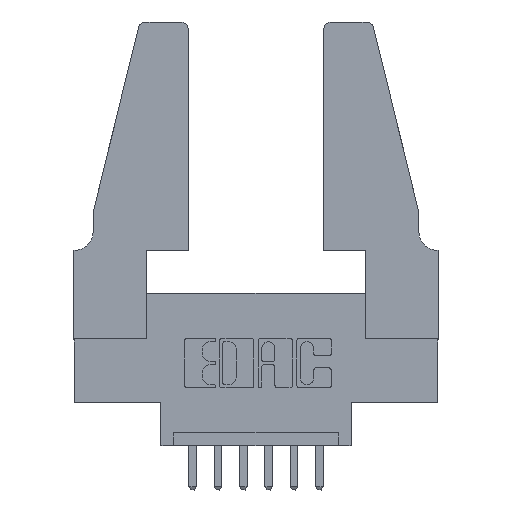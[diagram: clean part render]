
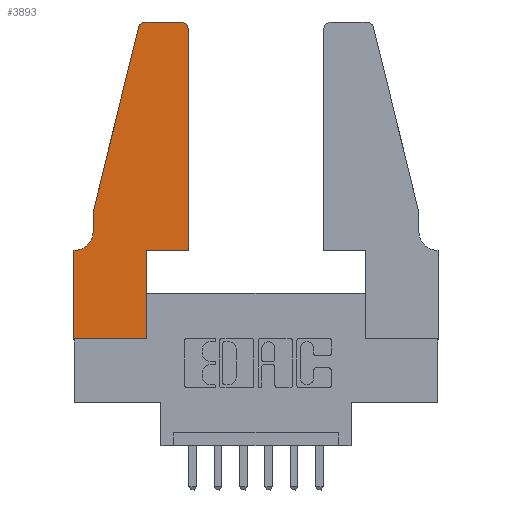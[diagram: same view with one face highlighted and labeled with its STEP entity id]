
A CAD part, top view. The second image highlights one B-rep face of the part: STEP entity #3893.
In plain terms, the highlighted planar face has unit normal (0, 0, 1).
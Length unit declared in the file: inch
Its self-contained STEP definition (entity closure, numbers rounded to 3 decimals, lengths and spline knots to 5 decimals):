
#195 = ORIENTED_EDGE ( 'NONE', *, *, #6748, .T. ) ;
#251 = AXIS2_PLACEMENT_3D ( 'NONE', #9541, #4079, #5767 ) ;
#274 = LINE ( 'NONE', #6401, #10389 ) ;
#316 = CARTESIAN_POINT ( 'NONE',  ( 0., 0., 0.37 ) ) ;
#455 = ORIENTED_EDGE ( 'NONE', *, *, #7087, .T. ) ;
#962 = EDGE_CURVE ( 'NONE', #7101, #1618, #11481, .T. ) ;
#1099 = CARTESIAN_POINT ( 'NONE',  ( 0.4505, 1.22, 0.37 ) ) ;
#1188 = ORIENTED_EDGE ( 'NONE', *, *, #3649, .T. ) ;
#1441 = VERTEX_POINT ( 'NONE', #6241 ) ;
#1507 = ORIENTED_EDGE ( 'NONE', *, *, #8306, .T. ) ;
#1570 = VECTOR ( 'NONE', #3611, 39.37008 ) ;
#1574 = DIRECTION ( 'NONE',  ( 1., 0., 0. ) ) ;
#1618 = VERTEX_POINT ( 'NONE', #7094 ) ;
#1653 = DIRECTION ( 'NONE',  ( -1., 0., 0. ) ) ;
#1662 = DIRECTION ( 'NONE',  ( 0., -1., 0. ) ) ;
#1713 = DIRECTION ( 'NONE',  ( 1., 0., 0. ) ) ;
#1851 = CARTESIAN_POINT ( 'NONE',  ( 0.0055, 0.35, 0.37 ) ) ;
#1860 = VECTOR ( 'NONE', #10426, 39.37008 ) ;
#1876 = ORIENTED_EDGE ( 'NONE', *, *, #962, .T. ) ;
#2293 = DIRECTION ( 'NONE',  ( 0., 0., -1. ) ) ;
#2810 = EDGE_CURVE ( 'NONE', #6537, #9482, #8172, .T. ) ;
#2836 = DIRECTION ( 'NONE',  ( 0., 1., 0. ) ) ;
#2928 = AXIS2_PLACEMENT_3D ( 'NONE', #3253, #2293, #9629 ) ;
#3149 = EDGE_CURVE ( 'NONE', #3715, #5302, #3883, .T. ) ;
#3253 = CARTESIAN_POINT ( 'NONE',  ( 0.0055, 0.42, 0.37 ) ) ;
#3288 = ORIENTED_EDGE ( 'NONE', *, *, #3149, .T. ) ;
#3290 = VERTEX_POINT ( 'NONE', #11260 ) ;
#3559 = CIRCLE ( 'NONE', #251, 0.03 ) ;
#3611 = DIRECTION ( 'NONE',  ( 1., 0., 0. ) ) ;
#3649 = EDGE_CURVE ( 'NONE', #5302, #11362, #4439, .T. ) ;
#3688 = VERTEX_POINT ( 'NONE', #9866 ) ;
#3715 = VERTEX_POINT ( 'NONE', #1851 ) ;
#3883 = LINE ( 'NONE', #7108, #10729 ) ;
#3893 = ADVANCED_FACE ( 'NONE', ( #6840 ), #5162, .T. ) ;
#3998 = VECTOR ( 'NONE', #1662, 39.37008 ) ;
#4022 = AXIS2_PLACEMENT_3D ( 'NONE', #5936, #10556, #6027 ) ;
#4079 = DIRECTION ( 'NONE',  ( 0., 0., 1. ) ) ;
#4189 = EDGE_CURVE ( 'NONE', #3290, #6929, #10902, .T. ) ;
#4343 = VERTEX_POINT ( 'NONE', #10335 ) ;
#4439 = LINE ( 'NONE', #6169, #3998 ) ;
#4602 = ORIENTED_EDGE ( 'NONE', *, *, #9904, .T. ) ;
#4687 = LINE ( 'NONE', #9246, #1860 ) ;
#5062 = LINE ( 'NONE', #6744, #11759 ) ;
#5162 = PLANE ( 'NONE',  #8461 ) ;
#5298 = CARTESIAN_POINT ( 'NONE',  ( 0., 0.35, 0.37 ) ) ;
#5302 = VERTEX_POINT ( 'NONE', #5298 ) ;
#5452 = ORIENTED_EDGE ( 'NONE', *, *, #4189, .T. ) ;
#5462 = CARTESIAN_POINT ( 'NONE',  ( 0.0755, 0.5, 0.37 ) ) ;
#5469 = CIRCLE ( 'NONE', #2928, 0.07 ) ;
#5507 = VECTOR ( 'NONE', #1713, 39.37008 ) ;
#5767 = DIRECTION ( 'NONE',  ( 1., 0., 0. ) ) ;
#5805 = LINE ( 'NONE', #7338, #1570 ) ;
#5930 = CARTESIAN_POINT ( 'NONE',  ( 0.4205, 1.25, 0.37 ) ) ;
#5936 = CARTESIAN_POINT ( 'NONE',  ( 0.4205, 1.22, 0.37 ) ) ;
#6002 = ORIENTED_EDGE ( 'NONE', *, *, #7707, .T. ) ;
#6027 = DIRECTION ( 'NONE',  ( 1., 0., 0. ) ) ;
#6089 = CARTESIAN_POINT ( 'NONE',  ( 0., 0.35, 0.37 ) ) ;
#6169 = CARTESIAN_POINT ( 'NONE',  ( 0., 0., 0.37 ) ) ;
#6241 = CARTESIAN_POINT ( 'NONE',  ( 0.284, 1.25, 0.37 ) ) ;
#6345 = ORIENTED_EDGE ( 'NONE', *, *, #2810, .T. ) ;
#6401 = CARTESIAN_POINT ( 'NONE',  ( 0.2605, 1.25, 0.37 ) ) ;
#6537 = VERTEX_POINT ( 'NONE', #1099 ) ;
#6744 = CARTESIAN_POINT ( 'NONE',  ( 0.0755, 0.5, 0.37 ) ) ;
#6748 = EDGE_CURVE ( 'NONE', #1441, #3688, #3559, .T. ) ;
#6840 = FACE_OUTER_BOUND ( 'NONE', #11246, .T. ) ;
#6929 = VERTEX_POINT ( 'NONE', #8174 ) ;
#7087 = EDGE_CURVE ( 'NONE', #4343, #6537, #4687, .T. ) ;
#7094 = CARTESIAN_POINT ( 'NONE',  ( 0.0755, 0.42, 0.37 ) ) ;
#7101 = VERTEX_POINT ( 'NONE', #8583 ) ;
#7108 = CARTESIAN_POINT ( 'NONE',  ( 0.0755, 0.35, 0.37 ) ) ;
#7211 = ORIENTED_EDGE ( 'NONE', *, *, #9388, .T. ) ;
#7338 = CARTESIAN_POINT ( 'NONE',  ( 0.4505, 0.35, 0.37 ) ) ;
#7401 = DIRECTION ( 'NONE',  ( -1., 0., 0. ) ) ;
#7696 = DIRECTION ( 'NONE',  ( -0.239, -0.971, 0. ) ) ;
#7707 = EDGE_CURVE ( 'NONE', #6929, #4343, #5805, .T. ) ;
#7888 = EDGE_CURVE ( 'NONE', #9482, #1441, #274, .T. ) ;
#8172 = CIRCLE ( 'NONE', #4022, 0.03 ) ;
#8174 = CARTESIAN_POINT ( 'NONE',  ( 0.2865, 0.35, 0.37 ) ) ;
#8306 = EDGE_CURVE ( 'NONE', #11362, #3290, #11782, .T. ) ;
#8461 = AXIS2_PLACEMENT_3D ( 'NONE', #6089, #8888, #1574 ) ;
#8583 = CARTESIAN_POINT ( 'NONE',  ( 0.0755, 0.5, 0.37 ) ) ;
#8888 = DIRECTION ( 'NONE',  ( 0., 0., 1. ) ) ;
#9081 = VECTOR ( 'NONE', #9971, 39.37008 ) ;
#9235 = CARTESIAN_POINT ( 'NONE',  ( 0.2865, 0.35, 0.37 ) ) ;
#9246 = CARTESIAN_POINT ( 'NONE',  ( 0.4505, 0.35, 0.37 ) ) ;
#9388 = EDGE_CURVE ( 'NONE', #1618, #3715, #5469, .T. ) ;
#9482 = VERTEX_POINT ( 'NONE', #5930 ) ;
#9541 = CARTESIAN_POINT ( 'NONE',  ( 0.284, 1.22, 0.37 ) ) ;
#9629 = DIRECTION ( 'NONE',  ( -1., 0., 0. ) ) ;
#9694 = CARTESIAN_POINT ( 'NONE',  ( 0., 0., 0.37 ) ) ;
#9866 = CARTESIAN_POINT ( 'NONE',  ( 0.25487, 1.22718, 0.37 ) ) ;
#9904 = EDGE_CURVE ( 'NONE', #3688, #7101, #5062, .T. ) ;
#9971 = DIRECTION ( 'NONE',  ( 0., -1., 0. ) ) ;
#10127 = ORIENTED_EDGE ( 'NONE', *, *, #7888, .T. ) ;
#10335 = CARTESIAN_POINT ( 'NONE',  ( 0.4505, 0.35, 0.37 ) ) ;
#10389 = VECTOR ( 'NONE', #7401, 39.37008 ) ;
#10426 = DIRECTION ( 'NONE',  ( 0., 1., 0. ) ) ;
#10556 = DIRECTION ( 'NONE',  ( 0., 0., 1. ) ) ;
#10729 = VECTOR ( 'NONE', #1653, 39.37008 ) ;
#10902 = LINE ( 'NONE', #9235, #11746 ) ;
#11246 = EDGE_LOOP ( 'NONE', ( #10127, #195, #4602, #1876, #7211, #3288, #1188, #1507, #5452, #6002, #455, #6345 ) ) ;
#11260 = CARTESIAN_POINT ( 'NONE',  ( 0.2865, 0., 0.37 ) ) ;
#11362 = VERTEX_POINT ( 'NONE', #316 ) ;
#11481 = LINE ( 'NONE', #5462, #9081 ) ;
#11746 = VECTOR ( 'NONE', #2836, 39.37008 ) ;
#11759 = VECTOR ( 'NONE', #7696, 39.37008 ) ;
#11782 = LINE ( 'NONE', #9694, #5507 ) ;
